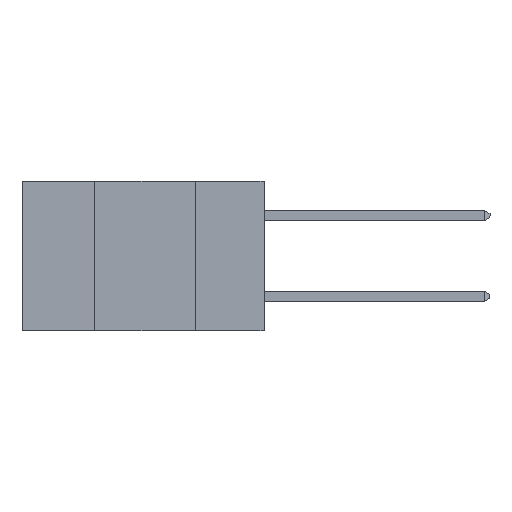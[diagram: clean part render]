
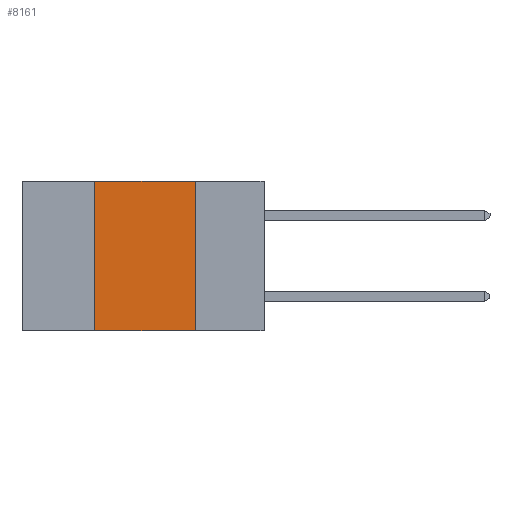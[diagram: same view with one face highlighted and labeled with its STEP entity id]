
A CAD part, left-side view. The second image highlights one B-rep face of the part: STEP entity #8161.
In plain terms, the highlighted planar face has unit normal (-1, 0, 0).
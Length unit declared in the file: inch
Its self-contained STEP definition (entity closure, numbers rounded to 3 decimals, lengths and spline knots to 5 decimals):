
#374 = VECTOR ( 'NONE', #11421, 39.37008 ) ;
#1565 = CARTESIAN_POINT ( 'NONE',  ( 0., 0.42, 0. ) ) ;
#2380 = VECTOR ( 'NONE', #8444, 39.37008 ) ;
#2592 = VERTEX_POINT ( 'NONE', #11503 ) ;
#4029 = EDGE_CURVE ( 'NONE', #9656, #2592, #12029, .T. ) ;
#4506 = VECTOR ( 'NONE', #14797, 39.37008 ) ;
#5328 = EDGE_CURVE ( 'NONE', #11556, #2592, #14721, .T. ) ;
#5728 = EDGE_CURVE ( 'NONE', #9656, #12583, #8991, .T. ) ;
#7196 = CARTESIAN_POINT ( 'NONE',  ( 0., 0.42, 0. ) ) ;
#7690 = VECTOR ( 'NONE', #17478, 39.37008 ) ;
#8161 = ADVANCED_FACE ( 'NONE', ( #15099 ), #12482, .F. ) ;
#8292 = CARTESIAN_POINT ( 'NONE',  ( 0., 0.6, 0. ) ) ;
#8444 = DIRECTION ( 'NONE',  ( 0., -1., 0. ) ) ;
#8991 = LINE ( 'NONE', #7196, #374 ) ;
#9181 = EDGE_CURVE ( 'NONE', #12583, #11556, #12861, .T. ) ;
#9656 = VERTEX_POINT ( 'NONE', #10950 ) ;
#9698 = DIRECTION ( 'NONE',  ( 0., 0., -1. ) ) ;
#10421 = CARTESIAN_POINT ( 'NONE',  ( 0., 0.6, -0.37 ) ) ;
#10950 = CARTESIAN_POINT ( 'NONE',  ( 0., 0.42, -0.37 ) ) ;
#11388 = ORIENTED_EDGE ( 'NONE', *, *, #5328, .F. ) ;
#11421 = DIRECTION ( 'NONE',  ( 0., 0., 1. ) ) ;
#11503 = CARTESIAN_POINT ( 'NONE',  ( 0., 0.17, -0.37 ) ) ;
#11556 = VERTEX_POINT ( 'NONE', #16626 ) ;
#11706 = ORIENTED_EDGE ( 'NONE', *, *, #9181, .F. ) ;
#12029 = LINE ( 'NONE', #10421, #4506 ) ;
#12482 = PLANE ( 'NONE',  #16499 ) ;
#12583 = VERTEX_POINT ( 'NONE', #1565 ) ;
#12696 = CARTESIAN_POINT ( 'NONE',  ( 0., 0.6, 0. ) ) ;
#12861 = LINE ( 'NONE', #12696, #2380 ) ;
#12938 = ORIENTED_EDGE ( 'NONE', *, *, #5728, .F. ) ;
#13023 = ORIENTED_EDGE ( 'NONE', *, *, #4029, .T. ) ;
#14721 = LINE ( 'NONE', #17933, #7690 ) ;
#14797 = DIRECTION ( 'NONE',  ( 0., -1., 0. ) ) ;
#15099 = FACE_OUTER_BOUND ( 'NONE', #16399, .T. ) ;
#16399 = EDGE_LOOP ( 'NONE', ( #11388, #11706, #12938, #13023 ) ) ;
#16499 = AXIS2_PLACEMENT_3D ( 'NONE', #8292, #18060, #9698 ) ;
#16626 = CARTESIAN_POINT ( 'NONE',  ( 0., 0.17, 0. ) ) ;
#17478 = DIRECTION ( 'NONE',  ( 0., 0., -1. ) ) ;
#17933 = CARTESIAN_POINT ( 'NONE',  ( 0., 0.17, 0. ) ) ;
#18060 = DIRECTION ( 'NONE',  ( 1., 0., 0. ) ) ;
